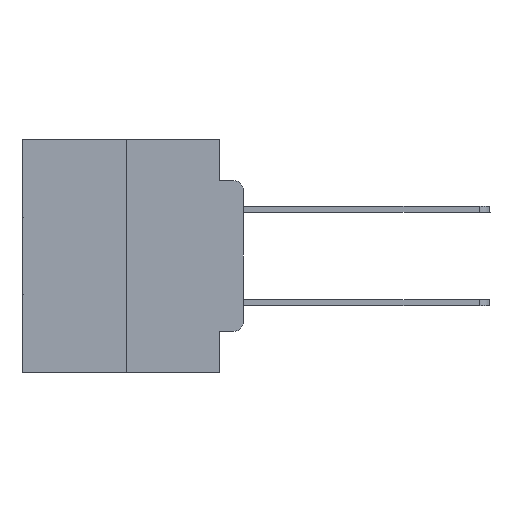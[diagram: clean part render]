
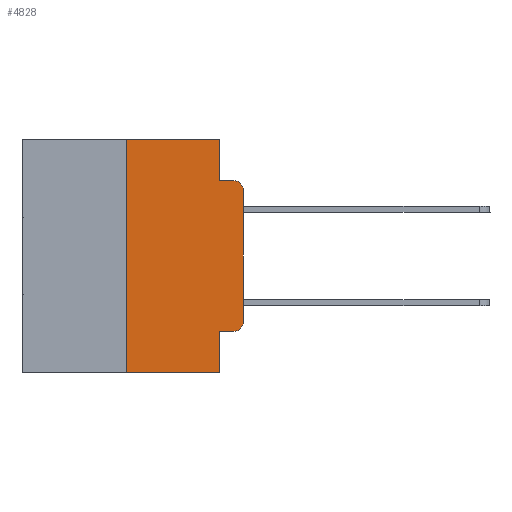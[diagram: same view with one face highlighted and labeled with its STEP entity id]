
A CAD part, left-side view. The second image highlights one B-rep face of the part: STEP entity #4828.
In plain terms, the highlighted planar face has unit normal (-1, 0, 0).
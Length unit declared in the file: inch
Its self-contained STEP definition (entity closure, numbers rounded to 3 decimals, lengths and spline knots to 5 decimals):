
#281 = EDGE_CURVE ( 'NONE', #13013, #5120, #20833, .T. ) ;
#351 = CARTESIAN_POINT ( 'NONE',  ( 0., 0.051, 0. ) ) ;
#496 = LINE ( 'NONE', #351, #17829 ) ;
#703 = VERTEX_POINT ( 'NONE', #8457 ) ;
#924 = EDGE_CURVE ( 'NONE', #11919, #13013, #2295, .T. ) ;
#1305 = ORIENTED_EDGE ( 'NONE', *, *, #4404, .T. ) ;
#1663 = EDGE_CURVE ( 'NONE', #9175, #5120, #1923, .T. ) ;
#1713 = EDGE_CURVE ( 'NONE', #12159, #5853, #11108, .T. ) ;
#1923 = LINE ( 'NONE', #15607, #20852 ) ;
#1938 = EDGE_CURVE ( 'NONE', #15155, #26889, #17398, .T. ) ;
#2295 = LINE ( 'NONE', #6631, #5393 ) ;
#2451 = CARTESIAN_POINT ( 'NONE',  ( 0., 0.051, 0. ) ) ;
#2876 = DIRECTION ( 'NONE',  ( 0., 0., -1. ) ) ;
#3236 = CARTESIAN_POINT ( 'NONE',  ( 0., 0., -0.1085 ) ) ;
#3379 = VECTOR ( 'NONE', #2876, 39.37008 ) ;
#3807 = AXIS2_PLACEMENT_3D ( 'NONE', #25335, #27723, #16342 ) ;
#4340 = CARTESIAN_POINT ( 'NONE',  ( 0., 0.25, -0.5 ) ) ;
#4404 = EDGE_CURVE ( 'NONE', #703, #11919, #13269, .T. ) ;
#4575 = VERTEX_POINT ( 'NONE', #19109 ) ;
#4663 = CARTESIAN_POINT ( 'NONE',  ( 0., 0.051, -0.0885 ) ) ;
#4673 = CARTESIAN_POINT ( 'NONE',  ( 0., 0.051, 0. ) ) ;
#4828 = ADVANCED_FACE ( 'NONE', ( #7000 ), #9423, .F. ) ;
#5120 = VERTEX_POINT ( 'NONE', #15097 ) ;
#5393 = VECTOR ( 'NONE', #27077, 39.37008 ) ;
#5433 = EDGE_CURVE ( 'NONE', #12159, #15155, #7403, .T. ) ;
#5853 = VERTEX_POINT ( 'NONE', #14301 ) ;
#6308 = EDGE_CURVE ( 'NONE', #4575, #5853, #496, .T. ) ;
#6631 = CARTESIAN_POINT ( 'NONE',  ( 0., 0., 0. ) ) ;
#6750 = DIRECTION ( 'NONE',  ( -1., 0., 0. ) ) ;
#6832 = CARTESIAN_POINT ( 'NONE',  ( 0., 0., -0.3915 ) ) ;
#7000 = FACE_OUTER_BOUND ( 'NONE', #9630, .T. ) ;
#7403 = LINE ( 'NONE', #24059, #25036 ) ;
#7838 = VECTOR ( 'NONE', #21588, 39.37008 ) ;
#7980 = DIRECTION ( 'NONE',  ( 0., 0., 1. ) ) ;
#8182 = DIRECTION ( 'NONE',  ( 0., -1., 0. ) ) ;
#8457 = CARTESIAN_POINT ( 'NONE',  ( 0., 0.02, -0.4115 ) ) ;
#8518 = CARTESIAN_POINT ( 'NONE',  ( 0., 0.25, 0. ) ) ;
#9175 = VERTEX_POINT ( 'NONE', #4663 ) ;
#9423 = PLANE ( 'NONE',  #3807 ) ;
#9532 = DIRECTION ( 'NONE',  ( 0., 0., -1. ) ) ;
#9534 = VECTOR ( 'NONE', #8182, 39.37008 ) ;
#9630 = EDGE_LOOP ( 'NONE', ( #17757, #15308, #21083, #21872, #21921, #10233, #14315, #17646, #16660, #1305 ) ) ;
#10233 = ORIENTED_EDGE ( 'NONE', *, *, #5433, .F. ) ;
#10651 = EDGE_CURVE ( 'NONE', #26889, #9175, #18859, .T. ) ;
#10925 = DIRECTION ( 'NONE',  ( 0., 0., -1. ) ) ;
#11108 = LINE ( 'NONE', #26665, #7838 ) ;
#11919 = VERTEX_POINT ( 'NONE', #6832 ) ;
#12159 = VERTEX_POINT ( 'NONE', #4340 ) ;
#12677 = VECTOR ( 'NONE', #26519, 39.37008 ) ;
#13013 = VERTEX_POINT ( 'NONE', #3236 ) ;
#13269 = CIRCLE ( 'NONE', #29070, 0.02 ) ;
#14301 = CARTESIAN_POINT ( 'NONE',  ( 0., 0.051, -0.5 ) ) ;
#14315 = ORIENTED_EDGE ( 'NONE', *, *, #1713, .T. ) ;
#15097 = CARTESIAN_POINT ( 'NONE',  ( 0., 0.02, -0.0885 ) ) ;
#15118 = CARTESIAN_POINT ( 'NONE',  ( 0., 0.02, -0.1085 ) ) ;
#15155 = VERTEX_POINT ( 'NONE', #8518 ) ;
#15308 = ORIENTED_EDGE ( 'NONE', *, *, #281, .T. ) ;
#15607 = CARTESIAN_POINT ( 'NONE',  ( 0., 0.051, -0.0885 ) ) ;
#15954 = DIRECTION ( 'NONE',  ( 0., 0., -1. ) ) ;
#16342 = DIRECTION ( 'NONE',  ( 0., 0., -1. ) ) ;
#16660 = ORIENTED_EDGE ( 'NONE', *, *, #19323, .T. ) ;
#17398 = LINE ( 'NONE', #20242, #12677 ) ;
#17646 = ORIENTED_EDGE ( 'NONE', *, *, #6308, .F. ) ;
#17757 = ORIENTED_EDGE ( 'NONE', *, *, #924, .T. ) ;
#17829 = VECTOR ( 'NONE', #9532, 39.37008 ) ;
#17851 = DIRECTION ( 'NONE',  ( -1., 0., 0. ) ) ;
#18859 = LINE ( 'NONE', #2451, #3379 ) ;
#19109 = CARTESIAN_POINT ( 'NONE',  ( 0., 0.051, -0.4115 ) ) ;
#19323 = EDGE_CURVE ( 'NONE', #4575, #703, #28757, .T. ) ;
#19647 = CARTESIAN_POINT ( 'NONE',  ( 0., 0.051, -0.4115 ) ) ;
#20242 = CARTESIAN_POINT ( 'NONE',  ( 0., 0.473, 0. ) ) ;
#20272 = DIRECTION ( 'NONE',  ( 0., -1., 0. ) ) ;
#20833 = CIRCLE ( 'NONE', #22709, 0.02 ) ;
#20852 = VECTOR ( 'NONE', #20272, 39.37008 ) ;
#21083 = ORIENTED_EDGE ( 'NONE', *, *, #1663, .F. ) ;
#21588 = DIRECTION ( 'NONE',  ( 0., -1., 0. ) ) ;
#21872 = ORIENTED_EDGE ( 'NONE', *, *, #10651, .F. ) ;
#21921 = ORIENTED_EDGE ( 'NONE', *, *, #1938, .F. ) ;
#22709 = AXIS2_PLACEMENT_3D ( 'NONE', #15118, #17851, #10925 ) ;
#24059 = CARTESIAN_POINT ( 'NONE',  ( 0., 0.25, 0. ) ) ;
#25036 = VECTOR ( 'NONE', #7980, 39.37008 ) ;
#25335 = CARTESIAN_POINT ( 'NONE',  ( 0., 0.473, 0. ) ) ;
#26519 = DIRECTION ( 'NONE',  ( 0., -1., 0. ) ) ;
#26665 = CARTESIAN_POINT ( 'NONE',  ( 0., 0.473, -0.5 ) ) ;
#26889 = VERTEX_POINT ( 'NONE', #4673 ) ;
#27077 = DIRECTION ( 'NONE',  ( 0., 0., 1. ) ) ;
#27723 = DIRECTION ( 'NONE',  ( 1., 0., 0. ) ) ;
#28757 = LINE ( 'NONE', #19647, #9534 ) ;
#29070 = AXIS2_PLACEMENT_3D ( 'NONE', #29445, #6750, #15954 ) ;
#29445 = CARTESIAN_POINT ( 'NONE',  ( 0., 0.02, -0.3915 ) ) ;
